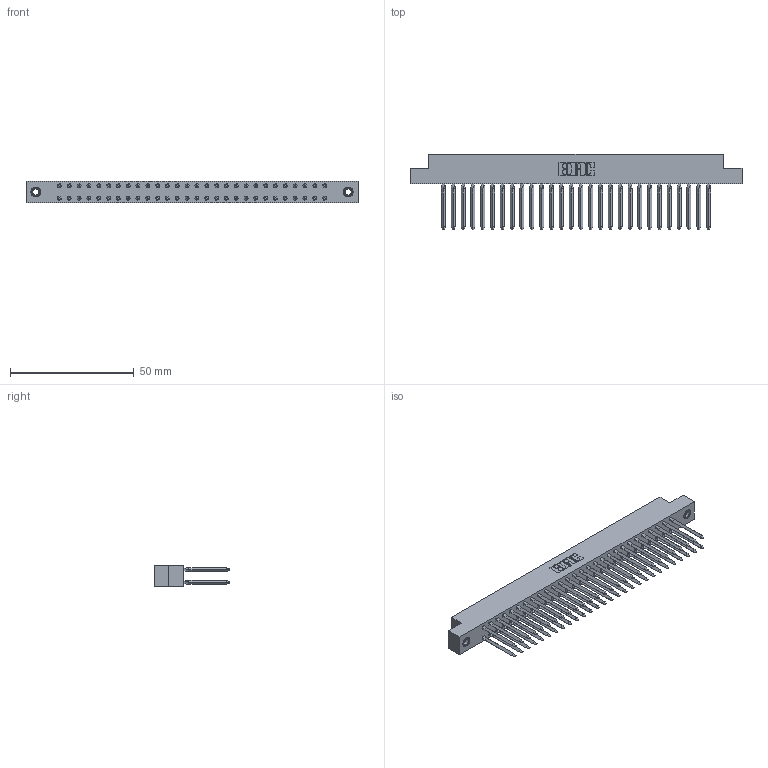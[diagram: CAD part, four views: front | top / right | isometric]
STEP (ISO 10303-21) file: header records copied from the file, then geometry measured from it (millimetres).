
FILE_DESCRIPTION (( 'STEP AP203' ), '1' );
FILE_NAME ('338-056-541-207.STEP', '2020-03-24T18:56:38', ( '' ), ( '' ), 'SwSTEP 2.0', 'SolidWorks 2016', '' );
FILE_SCHEMA (( 'CONFIG_CONTROL_DESIGN' ));
Length unit declared in the file: inch
Products named in the file (4): 338-290-001_541; 338-210-001_338-210-028-004; 345-250-001_345-250-005-103; 338-056-541-207
Assembly tree (59 placements, depth 2):
  338-056-541-207
    338-210-001_338-210-028-004
    338-290-001_541  x56
    345-250-001_345-250-005-103  x2
Bounding box: 133.96 x 30.56 x 8.71 mm (x, y, z)
Volume: 10342.4 mm3; surface area: 19527.7 mm2
Topology: 59 solids, 59 shells, 3906 faces, 10467 edges, 6634 vertices
Faces by surface type: plane 2714, cylinder 952, bspline 224, cone 12, torus 4
Entity records: 57193 total; most frequent: CARTESIAN_POINT 11283, ORIENTED_EDGE 9504, DIRECTION 8941, EDGE_CURVE 4752, VECTOR 3553, LINE 3553, VERTEX_POINT 3084, AXIS2_PLACEMENT_3D 2694
